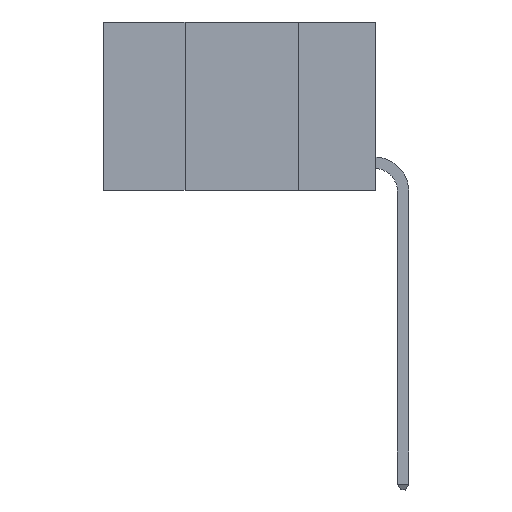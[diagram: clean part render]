
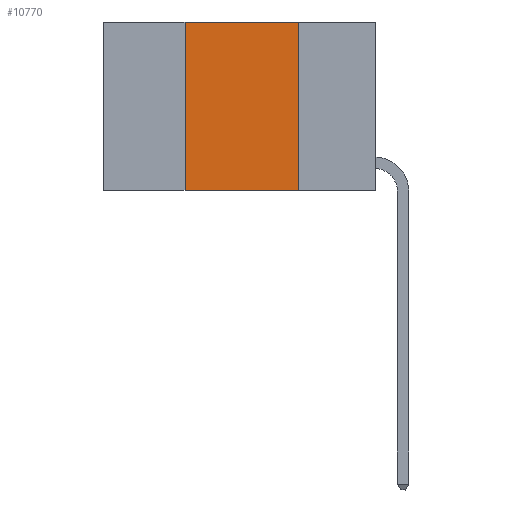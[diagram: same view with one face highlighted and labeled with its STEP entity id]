
A CAD part, left-side view. The second image highlights one B-rep face of the part: STEP entity #10770.
In plain terms, the highlighted planar face has unit normal (-1, 0, 0).
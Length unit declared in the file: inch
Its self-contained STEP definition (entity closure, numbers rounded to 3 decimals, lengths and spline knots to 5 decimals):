
#208 = EDGE_CURVE ( 'NONE', #12687, #19637, #5172, .T. ) ;
#470 = CARTESIAN_POINT ( 'NONE',  ( 0., 0.42, -0.37 ) ) ;
#612 = VERTEX_POINT ( 'NONE', #19163 ) ;
#2393 = CARTESIAN_POINT ( 'NONE',  ( 0., 0.42, 0. ) ) ;
#2791 = CARTESIAN_POINT ( 'NONE',  ( 0., 0.6, -0.37 ) ) ;
#4003 = VECTOR ( 'NONE', #12335, 39.37008 ) ;
#4444 = EDGE_CURVE ( 'NONE', #19637, #612, #6040, .T. ) ;
#5172 = LINE ( 'NONE', #11447, #16276 ) ;
#5392 = DIRECTION ( 'NONE',  ( 0., 0., -1. ) ) ;
#5599 = EDGE_LOOP ( 'NONE', ( #12342, #16447, #13723, #15511 ) ) ;
#5797 = LINE ( 'NONE', #2791, #17771 ) ;
#6040 = LINE ( 'NONE', #12124, #4003 ) ;
#6596 = CARTESIAN_POINT ( 'NONE',  ( 0., 0.6, 0. ) ) ;
#6896 = PLANE ( 'NONE',  #14911 ) ;
#8057 = DIRECTION ( 'NONE',  ( 0., 0., 1. ) ) ;
#9008 = EDGE_CURVE ( 'NONE', #612, #18501, #19295, .T. ) ;
#9794 = DIRECTION ( 'NONE',  ( 1., 0., 0. ) ) ;
#10770 = ADVANCED_FACE ( 'NONE', ( #19480 ), #6896, .F. ) ;
#11447 = CARTESIAN_POINT ( 'NONE',  ( 0., 0.42, 0. ) ) ;
#12124 = CARTESIAN_POINT ( 'NONE',  ( 0., 0.6, 0. ) ) ;
#12335 = DIRECTION ( 'NONE',  ( 0., -1., 0. ) ) ;
#12342 = ORIENTED_EDGE ( 'NONE', *, *, #9008, .F. ) ;
#12687 = VERTEX_POINT ( 'NONE', #470 ) ;
#12902 = DIRECTION ( 'NONE',  ( 0., 0., -1. ) ) ;
#13723 = ORIENTED_EDGE ( 'NONE', *, *, #208, .F. ) ;
#14911 = AXIS2_PLACEMENT_3D ( 'NONE', #6596, #9794, #12902 ) ;
#15511 = ORIENTED_EDGE ( 'NONE', *, *, #17299, .T. ) ;
#16276 = VECTOR ( 'NONE', #8057, 39.37008 ) ;
#16447 = ORIENTED_EDGE ( 'NONE', *, *, #4444, .F. ) ;
#16739 = CARTESIAN_POINT ( 'NONE',  ( 0., 0.17, -0.37 ) ) ;
#17299 = EDGE_CURVE ( 'NONE', #12687, #18501, #5797, .T. ) ;
#17771 = VECTOR ( 'NONE', #20122, 39.37008 ) ;
#18501 = VERTEX_POINT ( 'NONE', #16739 ) ;
#18866 = VECTOR ( 'NONE', #5392, 39.37008 ) ;
#19163 = CARTESIAN_POINT ( 'NONE',  ( 0., 0.17, 0. ) ) ;
#19295 = LINE ( 'NONE', #19506, #18866 ) ;
#19480 = FACE_OUTER_BOUND ( 'NONE', #5599, .T. ) ;
#19506 = CARTESIAN_POINT ( 'NONE',  ( 0., 0.17, 0. ) ) ;
#19637 = VERTEX_POINT ( 'NONE', #2393 ) ;
#20122 = DIRECTION ( 'NONE',  ( 0., -1., 0. ) ) ;
